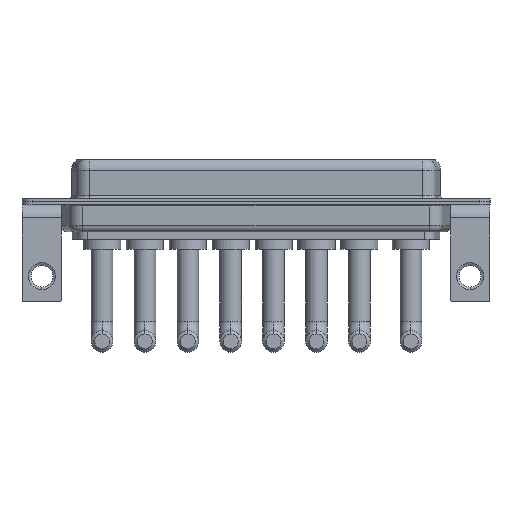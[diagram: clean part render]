
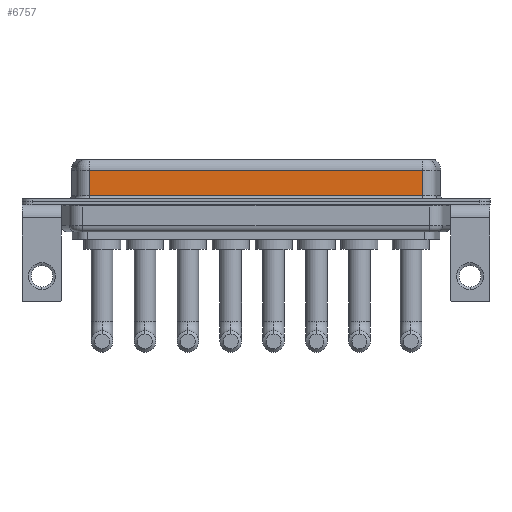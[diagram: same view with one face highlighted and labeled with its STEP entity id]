
A CAD part, front view. The second image highlights one B-rep face of the part: STEP entity #6757.
In plain terms, the highlighted planar face has unit normal (0, -1, 0).
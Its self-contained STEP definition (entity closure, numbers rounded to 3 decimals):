
#1045 = LINE ( 'NONE', #3237, #10777 ) ;
#1083 = VERTEX_POINT ( 'NONE', #6361 ) ;
#1740 = LINE ( 'NONE', #4782, #13185 ) ;
#2080 = DIRECTION ( 'NONE',  ( -1., 0., 0. ) ) ;
#2245 = EDGE_CURVE ( 'NONE', #11845, #10153, #11333, .T. ) ;
#2501 = DIRECTION ( 'NONE',  ( 1., 0., 0. ) ) ;
#2649 = VECTOR ( 'NONE', #2501, 1000. ) ;
#2841 = CARTESIAN_POINT ( 'NONE',  ( 56.462, -3.95, 4.65 ) ) ;
#3000 = CARTESIAN_POINT ( 'NONE',  ( 56.462, -3.95, 4.65 ) ) ;
#3237 = CARTESIAN_POINT ( 'NONE',  ( 7.038, -3.95, 6.4 ) ) ;
#3853 = DIRECTION ( 'NONE',  ( 0., 1., 0. ) ) ;
#4711 = FACE_OUTER_BOUND ( 'NONE', #11523, .T. ) ;
#4782 = CARTESIAN_POINT ( 'NONE',  ( 56.462, -3.95, 6.4 ) ) ;
#6361 = CARTESIAN_POINT ( 'NONE',  ( 7.038, -3.95, 4.65 ) ) ;
#6683 = EDGE_CURVE ( 'NONE', #8456, #10153, #1740, .T. ) ;
#6757 = ADVANCED_FACE ( 'NONE', ( #4711 ), #6855, .F. ) ;
#6855 = PLANE ( 'NONE',  #12042 ) ;
#7540 = ORIENTED_EDGE ( 'NONE', *, *, #2245, .T. ) ;
#7699 = ORIENTED_EDGE ( 'NONE', *, *, #6683, .F. ) ;
#7715 = CARTESIAN_POINT ( 'NONE',  ( 56.462, -3.95, 0.9 ) ) ;
#8456 = VERTEX_POINT ( 'NONE', #2841 ) ;
#8512 = LINE ( 'NONE', #3000, #11673 ) ;
#8878 = ORIENTED_EDGE ( 'NONE', *, *, #13867, .T. ) ;
#9731 = DIRECTION ( 'NONE',  ( 0., 0., -1. ) ) ;
#10153 = VERTEX_POINT ( 'NONE', #7715 ) ;
#10348 = DIRECTION ( 'NONE',  ( 0., 0., 1. ) ) ;
#10635 = CARTESIAN_POINT ( 'NONE',  ( 7.038, -3.95, 0.9 ) ) ;
#10777 = VECTOR ( 'NONE', #9731, 1000. ) ;
#11333 = LINE ( 'NONE', #12406, #2649 ) ;
#11406 = DIRECTION ( 'NONE',  ( 0., 0., -1. ) ) ;
#11523 = EDGE_LOOP ( 'NONE', ( #7699, #12624, #8878, #7540 ) ) ;
#11673 = VECTOR ( 'NONE', #2080, 1000. ) ;
#11845 = VERTEX_POINT ( 'NONE', #10635 ) ;
#11898 = EDGE_CURVE ( 'NONE', #8456, #1083, #8512, .T. ) ;
#12042 = AXIS2_PLACEMENT_3D ( 'NONE', #13401, #3853, #10348 ) ;
#12406 = CARTESIAN_POINT ( 'NONE',  ( 56.462, -3.95, 0.9 ) ) ;
#12624 = ORIENTED_EDGE ( 'NONE', *, *, #11898, .T. ) ;
#13185 = VECTOR ( 'NONE', #11406, 1000. ) ;
#13401 = CARTESIAN_POINT ( 'NONE',  ( 56.462, -3.95, 6.4 ) ) ;
#13867 = EDGE_CURVE ( 'NONE', #1083, #11845, #1045, .T. ) ;
